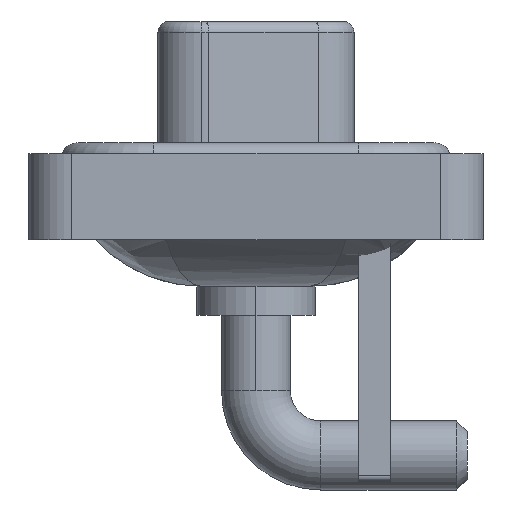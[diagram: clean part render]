
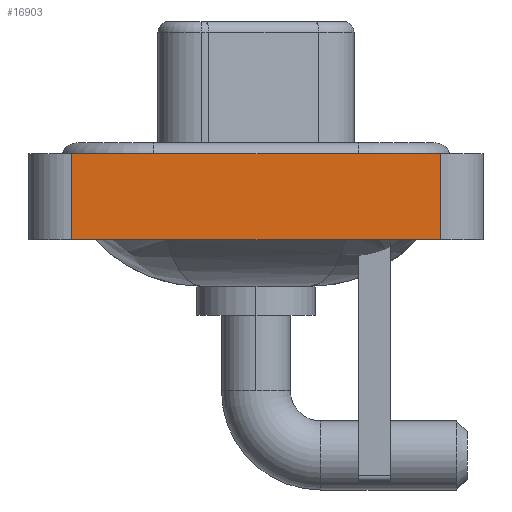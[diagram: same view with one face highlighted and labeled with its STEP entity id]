
A CAD part, left-side view. The second image highlights one B-rep face of the part: STEP entity #16903.
In plain terms, the highlighted planar face has unit normal (-1, 0, 0).
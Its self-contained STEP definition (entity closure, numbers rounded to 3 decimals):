
#86 = CARTESIAN_POINT ( 'NONE',  ( -7.35, -8.55, -3.6 ) ) ;
#177 = DIRECTION ( 'NONE',  ( 0., 0., 1. ) ) ;
#290 = VERTEX_POINT ( 'NONE', #15688 ) ;
#334 = ORIENTED_EDGE ( 'NONE', *, *, #13005, .F. ) ;
#525 = DIRECTION ( 'NONE',  ( 0., 0., 1. ) ) ;
#1421 = LINE ( 'NONE', #86, #5262 ) ;
#1826 = CARTESIAN_POINT ( 'NONE',  ( -7.35, -8.55, 0.4 ) ) ;
#2087 = DIRECTION ( 'NONE',  ( 0., 0., 1. ) ) ;
#2114 = VERTEX_POINT ( 'NONE', #3005 ) ;
#3005 = CARTESIAN_POINT ( 'NONE',  ( -7.35, -8.55, -3.6 ) ) ;
#3100 = EDGE_CURVE ( 'NONE', #290, #18131, #15049, .T. ) ;
#3279 = CARTESIAN_POINT ( 'NONE',  ( -7.35, -8.55, -3.6 ) ) ;
#5262 = VECTOR ( 'NONE', #177, 1000. ) ;
#8387 = VERTEX_POINT ( 'NONE', #13241 ) ;
#8432 = LINE ( 'NONE', #11079, #9992 ) ;
#9051 = EDGE_CURVE ( 'NONE', #8387, #2114, #8432, .T. ) ;
#9279 = LINE ( 'NONE', #15116, #18843 ) ;
#9368 = VECTOR ( 'NONE', #16281, 1000. ) ;
#9992 = VECTOR ( 'NONE', #17032, 1000. ) ;
#10487 = PLANE ( 'NONE',  #14014 ) ;
#10549 = ORIENTED_EDGE ( 'NONE', *, *, #3100, .F. ) ;
#11079 = CARTESIAN_POINT ( 'NONE',  ( -7.35, -8.55, -3.6 ) ) ;
#13005 = EDGE_CURVE ( 'NONE', #8387, #290, #9279, .T. ) ;
#13007 = ORIENTED_EDGE ( 'NONE', *, *, #17563, .T. ) ;
#13241 = CARTESIAN_POINT ( 'NONE',  ( -7.35, 8.55, -3.6 ) ) ;
#13618 = CARTESIAN_POINT ( 'NONE',  ( -7.35, -8.55, 0.4 ) ) ;
#14014 = AXIS2_PLACEMENT_3D ( 'NONE', #3279, #15089, #525 ) ;
#14276 = EDGE_LOOP ( 'NONE', ( #13007, #10549, #334, #17118 ) ) ;
#15049 = LINE ( 'NONE', #1826, #9368 ) ;
#15089 = DIRECTION ( 'NONE',  ( -1., 0., 0. ) ) ;
#15116 = CARTESIAN_POINT ( 'NONE',  ( -7.35, 8.55, -3.6 ) ) ;
#15688 = CARTESIAN_POINT ( 'NONE',  ( -7.35, 8.55, 0.4 ) ) ;
#16281 = DIRECTION ( 'NONE',  ( 0., -1., 0. ) ) ;
#16903 = ADVANCED_FACE ( 'NONE', ( #17865 ), #10487, .T. ) ;
#17032 = DIRECTION ( 'NONE',  ( 0., -1., 0. ) ) ;
#17118 = ORIENTED_EDGE ( 'NONE', *, *, #9051, .T. ) ;
#17563 = EDGE_CURVE ( 'NONE', #2114, #18131, #1421, .T. ) ;
#17865 = FACE_OUTER_BOUND ( 'NONE', #14276, .T. ) ;
#18131 = VERTEX_POINT ( 'NONE', #13618 ) ;
#18843 = VECTOR ( 'NONE', #2087, 1000. ) ;
